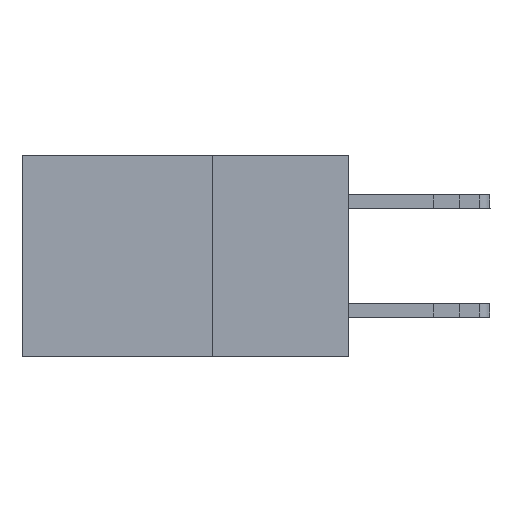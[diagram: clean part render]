
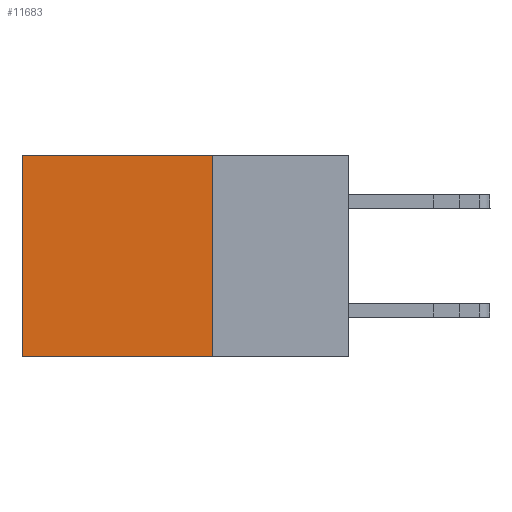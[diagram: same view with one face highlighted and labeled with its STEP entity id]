
A CAD part, left-side view. The second image highlights one B-rep face of the part: STEP entity #11683.
In plain terms, the highlighted planar face has unit normal (-1, 0, 0).
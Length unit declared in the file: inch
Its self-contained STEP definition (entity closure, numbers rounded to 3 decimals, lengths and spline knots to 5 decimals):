
#777 = VERTEX_POINT ( 'NONE', #10102 ) ;
#1035 = EDGE_CURVE ( 'NONE', #777, #1549, #5404, .T. ) ;
#1549 = VERTEX_POINT ( 'NONE', #6647 ) ;
#1976 = VECTOR ( 'NONE', #7554, 39.37008 ) ;
#2159 = VECTOR ( 'NONE', #12222, 39.37008 ) ;
#2720 = ORIENTED_EDGE ( 'NONE', *, *, #1035, .F. ) ;
#4142 = PLANE ( 'NONE',  #13949 ) ;
#4511 = LINE ( 'NONE', #8837, #17657 ) ;
#5404 = LINE ( 'NONE', #8104, #2159 ) ;
#5576 = ORIENTED_EDGE ( 'NONE', *, *, #6847, .T. ) ;
#6101 = ORIENTED_EDGE ( 'NONE', *, *, #14428, .T. ) ;
#6647 = CARTESIAN_POINT ( 'NONE',  ( 0.2615, 0.25, -0.37 ) ) ;
#6847 = EDGE_CURVE ( 'NONE', #777, #12172, #17251, .T. ) ;
#6946 = ORIENTED_EDGE ( 'NONE', *, *, #11351, .F. ) ;
#7554 = DIRECTION ( 'NONE',  ( 0., 1., 0. ) ) ;
#8104 = CARTESIAN_POINT ( 'NONE',  ( 0.2615, 0.25, -0.37 ) ) ;
#8246 = VECTOR ( 'NONE', #11926, 39.37008 ) ;
#8285 = DIRECTION ( 'NONE',  ( 0., 0., -1. ) ) ;
#8555 = EDGE_LOOP ( 'NONE', ( #6101, #6946, #2720, #5576 ) ) ;
#8837 = CARTESIAN_POINT ( 'NONE',  ( 0.2615, 0.25, -0.37 ) ) ;
#8891 = CARTESIAN_POINT ( 'NONE',  ( 0.2615, 0.6, -0.37 ) ) ;
#9275 = CARTESIAN_POINT ( 'NONE',  ( 0.2615, 0.25, 0. ) ) ;
#9637 = CARTESIAN_POINT ( 'NONE',  ( 0.2615, 0.25, -0.37 ) ) ;
#10102 = CARTESIAN_POINT ( 'NONE',  ( 0.2615, 0.25, 0. ) ) ;
#11351 = EDGE_CURVE ( 'NONE', #1549, #15820, #4511, .T. ) ;
#11435 = DIRECTION ( 'NONE',  ( 0., 1., 0. ) ) ;
#11683 = ADVANCED_FACE ( 'NONE', ( #15179 ), #4142, .F. ) ;
#11926 = DIRECTION ( 'NONE',  ( 0., 0., -1. ) ) ;
#12172 = VERTEX_POINT ( 'NONE', #12985 ) ;
#12222 = DIRECTION ( 'NONE',  ( 0., 0., -1. ) ) ;
#12985 = CARTESIAN_POINT ( 'NONE',  ( 0.2615, 0.6, 0. ) ) ;
#13949 = AXIS2_PLACEMENT_3D ( 'NONE', #9637, #15089, #8285 ) ;
#14428 = EDGE_CURVE ( 'NONE', #12172, #15820, #14437, .T. ) ;
#14437 = LINE ( 'NONE', #14524, #8246 ) ;
#14524 = CARTESIAN_POINT ( 'NONE',  ( 0.2615, 0.6, -0.37 ) ) ;
#15089 = DIRECTION ( 'NONE',  ( 1., 0., 0. ) ) ;
#15179 = FACE_OUTER_BOUND ( 'NONE', #8555, .T. ) ;
#15820 = VERTEX_POINT ( 'NONE', #8891 ) ;
#17251 = LINE ( 'NONE', #9275, #1976 ) ;
#17657 = VECTOR ( 'NONE', #11435, 39.37008 ) ;
